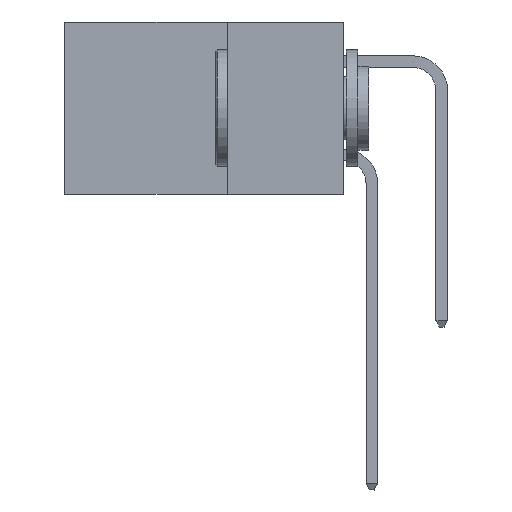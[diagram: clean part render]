
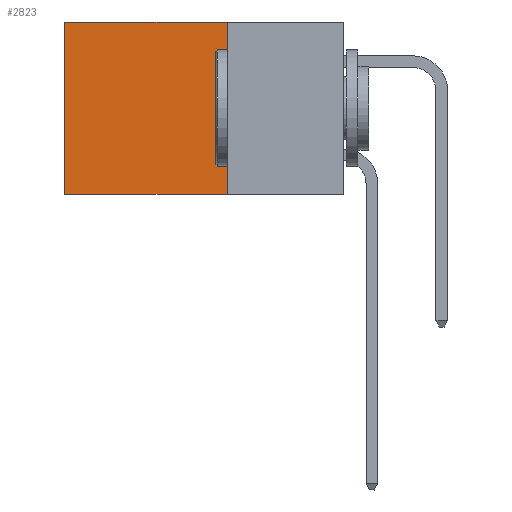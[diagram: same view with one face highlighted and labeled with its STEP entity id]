
A CAD part, left-side view. The second image highlights one B-rep face of the part: STEP entity #2823.
In plain terms, the highlighted planar face has unit normal (-1, 0, 0).
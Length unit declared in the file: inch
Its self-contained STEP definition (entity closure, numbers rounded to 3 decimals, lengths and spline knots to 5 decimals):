
#524 = CARTESIAN_POINT ( 'NONE',  ( 0.298, 0.25, 0. ) ) ;
#572 = EDGE_CURVE ( 'NONE', #11875, #2412, #9881, .T. ) ;
#1198 = VECTOR ( 'NONE', #10020, 39.37008 ) ;
#1517 = LINE ( 'NONE', #4471, #1198 ) ;
#1608 = CARTESIAN_POINT ( 'NONE',  ( 0.298, 0.6, 0. ) ) ;
#1681 = VERTEX_POINT ( 'NONE', #9594 ) ;
#1684 = FACE_OUTER_BOUND ( 'NONE', #3834, .T. ) ;
#1921 = LINE ( 'NONE', #1608, #6869 ) ;
#2025 = AXIS2_PLACEMENT_3D ( 'NONE', #3695, #4095, #4249 ) ;
#2100 = CARTESIAN_POINT ( 'NONE',  ( 0.298, 0.25, -0.37 ) ) ;
#2176 = LINE ( 'NONE', #2100, #4309 ) ;
#2394 = VERTEX_POINT ( 'NONE', #6110 ) ;
#2412 = VERTEX_POINT ( 'NONE', #11368 ) ;
#2446 = ORIENTED_EDGE ( 'NONE', *, *, #8195, .T. ) ;
#2459 = ORIENTED_EDGE ( 'NONE', *, *, #11395, .F. ) ;
#2471 = ORIENTED_EDGE ( 'NONE', *, *, #572, .F. ) ;
#2484 = ORIENTED_EDGE ( 'NONE', *, *, #4384, .T. ) ;
#2652 = DIRECTION ( 'NONE',  ( 0., 0., -1. ) ) ;
#2739 = CARTESIAN_POINT ( 'NONE',  ( 0.298, 0.25, 0. ) ) ;
#2823 = ADVANCED_FACE ( 'NONE', ( #1684 ), #4111, .F. ) ;
#3695 = CARTESIAN_POINT ( 'NONE',  ( 0.298, 0.25, 0. ) ) ;
#3800 = DIRECTION ( 'NONE',  ( 0., 0., -1. ) ) ;
#3834 = EDGE_LOOP ( 'NONE', ( #2446, #2459, #2471, #2484 ) ) ;
#4095 = DIRECTION ( 'NONE',  ( 1., 0., 0. ) ) ;
#4111 = PLANE ( 'NONE',  #2025 ) ;
#4249 = DIRECTION ( 'NONE',  ( 0., 0., -1. ) ) ;
#4309 = VECTOR ( 'NONE', #7015, 39.37008 ) ;
#4384 = EDGE_CURVE ( 'NONE', #11875, #1681, #1517, .T. ) ;
#4471 = CARTESIAN_POINT ( 'NONE',  ( 0.298, 0.25, 0. ) ) ;
#6110 = CARTESIAN_POINT ( 'NONE',  ( 0.298, 0.6, -0.37 ) ) ;
#6869 = VECTOR ( 'NONE', #2652, 39.37008 ) ;
#7015 = DIRECTION ( 'NONE',  ( 0., 1., 0. ) ) ;
#8195 = EDGE_CURVE ( 'NONE', #1681, #2394, #1921, .T. ) ;
#9594 = CARTESIAN_POINT ( 'NONE',  ( 0.298, 0.6, 0. ) ) ;
#9881 = LINE ( 'NONE', #2739, #11997 ) ;
#10020 = DIRECTION ( 'NONE',  ( 0., 1., 0. ) ) ;
#11368 = CARTESIAN_POINT ( 'NONE',  ( 0.298, 0.25, -0.37 ) ) ;
#11395 = EDGE_CURVE ( 'NONE', #2412, #2394, #2176, .T. ) ;
#11875 = VERTEX_POINT ( 'NONE', #524 ) ;
#11997 = VECTOR ( 'NONE', #3800, 39.37008 ) ;
